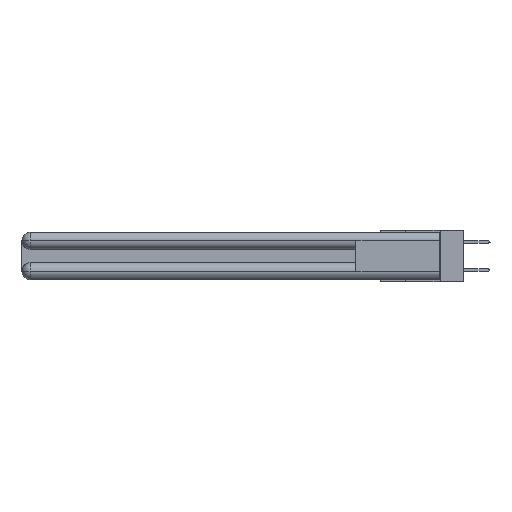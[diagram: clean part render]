
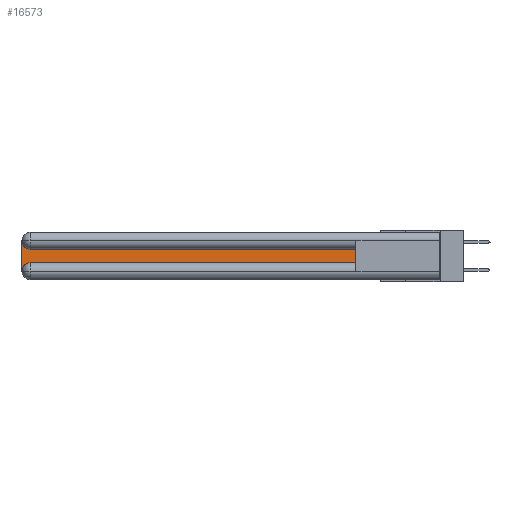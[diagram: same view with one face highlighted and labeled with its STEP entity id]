
A CAD part, left-side view. The second image highlights one B-rep face of the part: STEP entity #16573.
In plain terms, the highlighted planar face has unit normal (-1, 0, 0).
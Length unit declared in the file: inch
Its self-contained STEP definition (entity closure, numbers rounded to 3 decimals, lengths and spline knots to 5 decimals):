
#735 = AXIS2_PLACEMENT_3D ( 'NONE', #27451, #11693, #6473 ) ;
#2039 = CARTESIAN_POINT ( 'NONE',  ( 0.075, 0.6, -0.2175 ) ) ;
#2191 = CARTESIAN_POINT ( 'NONE',  ( 0.075, 3., -0.1225 ) ) ;
#2197 = VERTEX_POINT ( 'NONE', #3847 ) ;
#2456 = EDGE_CURVE ( 'NONE', #30127, #2197, #19239, .T. ) ;
#3021 = ORIENTED_EDGE ( 'NONE', *, *, #2456, .T. ) ;
#3203 = LINE ( 'NONE', #3287, #34732 ) ;
#3287 = CARTESIAN_POINT ( 'NONE',  ( 0.075, 0.6, -0.2175 ) ) ;
#3312 = CARTESIAN_POINT ( 'NONE',  ( 0.075, 2.94, -0.2775 ) ) ;
#3847 = CARTESIAN_POINT ( 'NONE',  ( 0.075, 0.6, -0.1225 ) ) ;
#4005 = CARTESIAN_POINT ( 'NONE',  ( 0.075, 3., -0.0625 ) ) ;
#4814 = DIRECTION ( 'NONE',  ( 0., 0., 1. ) ) ;
#5403 = ORIENTED_EDGE ( 'NONE', *, *, #12393, .T. ) ;
#5953 = DIRECTION ( 'NONE',  ( 1., 0., 0. ) ) ;
#6044 = VECTOR ( 'NONE', #17231, 39.37008 ) ;
#6473 = DIRECTION ( 'NONE',  ( 0., 0., -1. ) ) ;
#6493 = EDGE_CURVE ( 'NONE', #19467, #30127, #3203, .T. ) ;
#6714 = EDGE_CURVE ( 'NONE', #27425, #19169, #34693, .T. ) ;
#6925 = CIRCLE ( 'NONE', #735, 0.06 ) ;
#8573 = CARTESIAN_POINT ( 'NONE',  ( 0.075, 0.6, -0.2175 ) ) ;
#9956 = CIRCLE ( 'NONE', #24362, 0.06 ) ;
#10001 = PLANE ( 'NONE',  #27390 ) ;
#11693 = DIRECTION ( 'NONE',  ( 1., 0., 0. ) ) ;
#12393 = EDGE_CURVE ( 'NONE', #2197, #30958, #14769, .T. ) ;
#14509 = CARTESIAN_POINT ( 'NONE',  ( 0.075, 3., -0.2175 ) ) ;
#14769 = LINE ( 'NONE', #31305, #28253 ) ;
#15625 = VECTOR ( 'NONE', #4814, 39.37008 ) ;
#16482 = CARTESIAN_POINT ( 'NONE',  ( 0.075, 3., -0.2775 ) ) ;
#16573 = ADVANCED_FACE ( 'NONE', ( #20893 ), #10001, .F. ) ;
#17231 = DIRECTION ( 'NONE',  ( 0., 0., -1. ) ) ;
#17253 = ORIENTED_EDGE ( 'NONE', *, *, #23395, .T. ) ;
#17911 = DIRECTION ( 'NONE',  ( 0., 1., 0. ) ) ;
#19169 = VERTEX_POINT ( 'NONE', #16482 ) ;
#19239 = LINE ( 'NONE', #2039, #15625 ) ;
#19467 = VERTEX_POINT ( 'NONE', #31753 ) ;
#20893 = FACE_OUTER_BOUND ( 'NONE', #29266, .T. ) ;
#23395 = EDGE_CURVE ( 'NONE', #19169, #19467, #9956, .T. ) ;
#24023 = EDGE_CURVE ( 'NONE', #30958, #27425, #6925, .T. ) ;
#24362 = AXIS2_PLACEMENT_3D ( 'NONE', #3312, #5953, #27838 ) ;
#25790 = ORIENTED_EDGE ( 'NONE', *, *, #24023, .T. ) ;
#26494 = ORIENTED_EDGE ( 'NONE', *, *, #6493, .T. ) ;
#27280 = ORIENTED_EDGE ( 'NONE', *, *, #6714, .T. ) ;
#27390 = AXIS2_PLACEMENT_3D ( 'NONE', #2191, #28617, #34009 ) ;
#27425 = VERTEX_POINT ( 'NONE', #4005 ) ;
#27451 = CARTESIAN_POINT ( 'NONE',  ( 0.075, 2.94, -0.0625 ) ) ;
#27838 = DIRECTION ( 'NONE',  ( 0., 0., -1. ) ) ;
#28253 = VECTOR ( 'NONE', #17911, 39.37008 ) ;
#28554 = CARTESIAN_POINT ( 'NONE',  ( 0.075, 2.94, -0.1225 ) ) ;
#28617 = DIRECTION ( 'NONE',  ( 1., 0., 0. ) ) ;
#29266 = EDGE_LOOP ( 'NONE', ( #5403, #25790, #27280, #17253, #26494, #3021 ) ) ;
#30127 = VERTEX_POINT ( 'NONE', #8573 ) ;
#30958 = VERTEX_POINT ( 'NONE', #28554 ) ;
#31305 = CARTESIAN_POINT ( 'NONE',  ( 0.075, 0.6, -0.1225 ) ) ;
#31753 = CARTESIAN_POINT ( 'NONE',  ( 0.075, 2.94, -0.2175 ) ) ;
#32848 = DIRECTION ( 'NONE',  ( 0., -1., 0. ) ) ;
#34009 = DIRECTION ( 'NONE',  ( 0., 0., -1. ) ) ;
#34693 = LINE ( 'NONE', #14509, #6044 ) ;
#34732 = VECTOR ( 'NONE', #32848, 39.37008 ) ;
